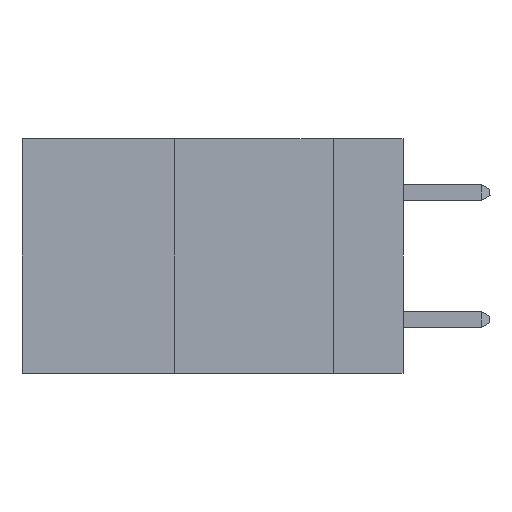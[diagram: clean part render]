
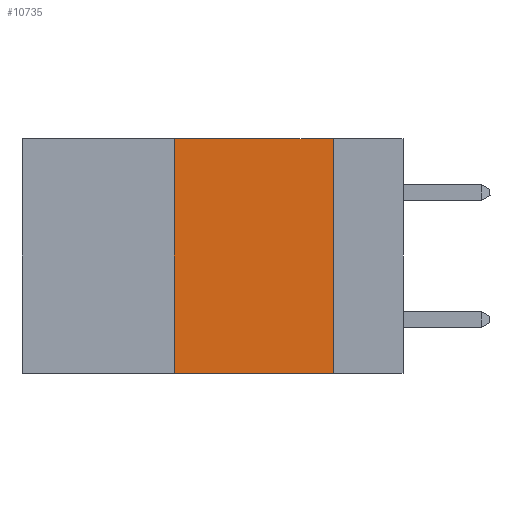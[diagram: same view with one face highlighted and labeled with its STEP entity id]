
A CAD part, left-side view. The second image highlights one B-rep face of the part: STEP entity #10735.
In plain terms, the highlighted planar face has unit normal (-1, 0, 0).
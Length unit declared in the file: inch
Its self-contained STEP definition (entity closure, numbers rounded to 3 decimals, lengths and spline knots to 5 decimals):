
#63 = CARTESIAN_POINT ( 'NONE',  ( 0., 0.6, 0. ) ) ;
#69 = EDGE_CURVE ( 'NONE', #18024, #9505, #15662, .T. ) ;
#182 = CARTESIAN_POINT ( 'NONE',  ( 0., 0.36, 0. ) ) ;
#212 = EDGE_CURVE ( 'NONE', #8038, #18024, #9854, .T. ) ;
#781 = CARTESIAN_POINT ( 'NONE',  ( 0., 0.6, 0. ) ) ;
#882 = DIRECTION ( 'NONE',  ( 0., 0., -1. ) ) ;
#2759 = VECTOR ( 'NONE', #3411, 39.37008 ) ;
#3032 = AXIS2_PLACEMENT_3D ( 'NONE', #781, #10294, #882 ) ;
#3411 = DIRECTION ( 'NONE',  ( 0., -1., 0. ) ) ;
#3670 = VECTOR ( 'NONE', #17321, 39.37008 ) ;
#4303 = CARTESIAN_POINT ( 'NONE',  ( 0., 0.11, 0. ) ) ;
#5463 = PLANE ( 'NONE',  #3032 ) ;
#5759 = CARTESIAN_POINT ( 'NONE',  ( 0., 0.36, 0. ) ) ;
#5784 = ORIENTED_EDGE ( 'NONE', *, *, #13889, .F. ) ;
#7178 = ORIENTED_EDGE ( 'NONE', *, *, #69, .F. ) ;
#8038 = VERTEX_POINT ( 'NONE', #16604 ) ;
#8273 = VERTEX_POINT ( 'NONE', #17692 ) ;
#9505 = VERTEX_POINT ( 'NONE', #4303 ) ;
#9699 = ORIENTED_EDGE ( 'NONE', *, *, #212, .F. ) ;
#9854 = LINE ( 'NONE', #5759, #17289 ) ;
#10006 = CARTESIAN_POINT ( 'NONE',  ( 0., 0.6, -0.37 ) ) ;
#10294 = DIRECTION ( 'NONE',  ( 1., 0., 0. ) ) ;
#10735 = ADVANCED_FACE ( 'NONE', ( #13382 ), #5463, .F. ) ;
#11724 = DIRECTION ( 'NONE',  ( 0., 0., 1. ) ) ;
#11894 = EDGE_CURVE ( 'NONE', #8038, #8273, #17880, .T. ) ;
#12440 = VECTOR ( 'NONE', #20232, 39.37008 ) ;
#12547 = CARTESIAN_POINT ( 'NONE',  ( 0., 0.11, 0. ) ) ;
#13382 = FACE_OUTER_BOUND ( 'NONE', #18653, .T. ) ;
#13889 = EDGE_CURVE ( 'NONE', #9505, #8273, #15859, .T. ) ;
#14749 = ORIENTED_EDGE ( 'NONE', *, *, #11894, .T. ) ;
#15662 = LINE ( 'NONE', #63, #3670 ) ;
#15859 = LINE ( 'NONE', #12547, #12440 ) ;
#16604 = CARTESIAN_POINT ( 'NONE',  ( 0., 0.36, -0.37 ) ) ;
#17289 = VECTOR ( 'NONE', #11724, 39.37008 ) ;
#17321 = DIRECTION ( 'NONE',  ( 0., -1., 0. ) ) ;
#17692 = CARTESIAN_POINT ( 'NONE',  ( 0., 0.11, -0.37 ) ) ;
#17880 = LINE ( 'NONE', #10006, #2759 ) ;
#18024 = VERTEX_POINT ( 'NONE', #182 ) ;
#18653 = EDGE_LOOP ( 'NONE', ( #5784, #7178, #9699, #14749 ) ) ;
#20232 = DIRECTION ( 'NONE',  ( 0., 0., -1. ) ) ;
